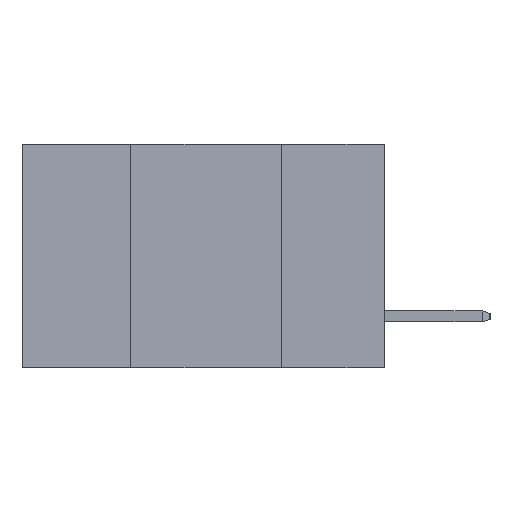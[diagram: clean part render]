
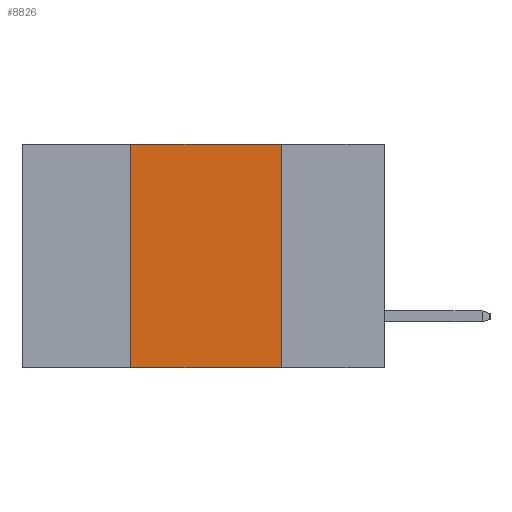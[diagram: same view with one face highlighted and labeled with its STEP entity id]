
A CAD part, left-side view. The second image highlights one B-rep face of the part: STEP entity #8826.
In plain terms, the highlighted planar face has unit normal (-1, 0, 0).
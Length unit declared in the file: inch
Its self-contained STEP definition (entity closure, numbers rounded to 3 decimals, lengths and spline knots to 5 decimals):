
#381 = LINE ( 'NONE', #12356, #4960 ) ;
#466 = VERTEX_POINT ( 'NONE', #12809 ) ;
#1051 = DIRECTION ( 'NONE',  ( 0., 0., -1. ) ) ;
#1310 = PLANE ( 'NONE',  #8234 ) ;
#2130 = CARTESIAN_POINT ( 'NONE',  ( 0., 0.42, -0.37 ) ) ;
#2489 = DIRECTION ( 'NONE',  ( 0., 0., -1. ) ) ;
#3170 = VERTEX_POINT ( 'NONE', #2130 ) ;
#3239 = CARTESIAN_POINT ( 'NONE',  ( 0., 0.42, 0. ) ) ;
#4431 = VECTOR ( 'NONE', #1051, 39.37008 ) ;
#4960 = VECTOR ( 'NONE', #8331, 39.37008 ) ;
#5087 = VERTEX_POINT ( 'NONE', #5100 ) ;
#5100 = CARTESIAN_POINT ( 'NONE',  ( 0., 0.17, -0.37 ) ) ;
#5143 = VECTOR ( 'NONE', #12375, 39.37008 ) ;
#5338 = EDGE_LOOP ( 'NONE', ( #7036, #7353, #10078, #10714 ) ) ;
#6470 = VECTOR ( 'NONE', #9487, 39.37008 ) ;
#7036 = ORIENTED_EDGE ( 'NONE', *, *, #10875, .F. ) ;
#7215 = CARTESIAN_POINT ( 'NONE',  ( 0., 0.17, 0. ) ) ;
#7353 = ORIENTED_EDGE ( 'NONE', *, *, #10124, .F. ) ;
#7562 = CARTESIAN_POINT ( 'NONE',  ( 0., 0.17, 0. ) ) ;
#7604 = LINE ( 'NONE', #11461, #5143 ) ;
#8234 = AXIS2_PLACEMENT_3D ( 'NONE', #12735, #8799, #2489 ) ;
#8331 = DIRECTION ( 'NONE',  ( 0., -1., 0. ) ) ;
#8799 = DIRECTION ( 'NONE',  ( 1., 0., 0. ) ) ;
#8826 = ADVANCED_FACE ( 'NONE', ( #10822 ), #1310, .F. ) ;
#9487 = DIRECTION ( 'NONE',  ( 0., 0., 1. ) ) ;
#9488 = LINE ( 'NONE', #3239, #6470 ) ;
#9494 = EDGE_CURVE ( 'NONE', #3170, #5087, #7604, .T. ) ;
#10078 = ORIENTED_EDGE ( 'NONE', *, *, #10203, .F. ) ;
#10124 = EDGE_CURVE ( 'NONE', #466, #10689, #381, .T. ) ;
#10203 = EDGE_CURVE ( 'NONE', #3170, #466, #9488, .T. ) ;
#10689 = VERTEX_POINT ( 'NONE', #7215 ) ;
#10714 = ORIENTED_EDGE ( 'NONE', *, *, #9494, .T. ) ;
#10760 = LINE ( 'NONE', #7562, #4431 ) ;
#10822 = FACE_OUTER_BOUND ( 'NONE', #5338, .T. ) ;
#10875 = EDGE_CURVE ( 'NONE', #10689, #5087, #10760, .T. ) ;
#11461 = CARTESIAN_POINT ( 'NONE',  ( 0., 0.6, -0.37 ) ) ;
#12356 = CARTESIAN_POINT ( 'NONE',  ( 0., 0.6, 0. ) ) ;
#12375 = DIRECTION ( 'NONE',  ( 0., -1., 0. ) ) ;
#12735 = CARTESIAN_POINT ( 'NONE',  ( 0., 0.6, 0. ) ) ;
#12809 = CARTESIAN_POINT ( 'NONE',  ( 0., 0.42, 0. ) ) ;
